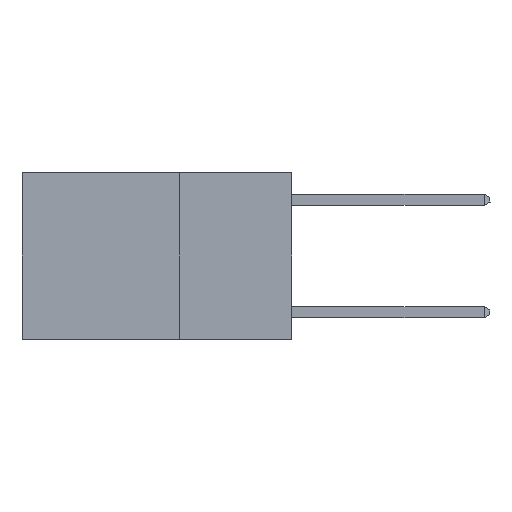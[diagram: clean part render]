
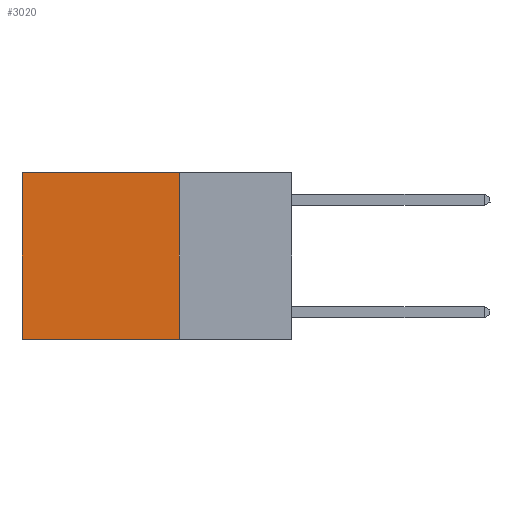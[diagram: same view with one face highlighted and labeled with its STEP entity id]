
A CAD part, left-side view. The second image highlights one B-rep face of the part: STEP entity #3020.
In plain terms, the highlighted planar face has unit normal (-1, 0, 0).
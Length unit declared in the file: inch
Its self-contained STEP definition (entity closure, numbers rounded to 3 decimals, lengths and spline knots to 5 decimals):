
#401 = EDGE_CURVE ( 'NONE', #8646, #3516, #3455, .T. ) ;
#670 = ORIENTED_EDGE ( 'NONE', *, *, #8644, .F. ) ;
#1688 = ORIENTED_EDGE ( 'NONE', *, *, #6867, .F. ) ;
#1991 = DIRECTION ( 'NONE',  ( 0., 1., 0. ) ) ;
#2136 = LINE ( 'NONE', #8721, #4109 ) ;
#2543 = DIRECTION ( 'NONE',  ( 0., 1., 0. ) ) ;
#3020 = ADVANCED_FACE ( 'NONE', ( #8531 ), #8884, .F. ) ;
#3200 = VECTOR ( 'NONE', #3690, 39.37008 ) ;
#3455 = LINE ( 'NONE', #4082, #3200 ) ;
#3516 = VERTEX_POINT ( 'NONE', #9144 ) ;
#3690 = DIRECTION ( 'NONE',  ( 0., 0., -1. ) ) ;
#3838 = ORIENTED_EDGE ( 'NONE', *, *, #5899, .T. ) ;
#3918 = ORIENTED_EDGE ( 'NONE', *, *, #401, .T. ) ;
#4082 = CARTESIAN_POINT ( 'NONE',  ( 0.2625, 0.6, 0. ) ) ;
#4109 = VECTOR ( 'NONE', #1991, 39.37008 ) ;
#4309 = LINE ( 'NONE', #10726, #6837 ) ;
#5013 = CARTESIAN_POINT ( 'NONE',  ( 0.2625, 0.25, 0. ) ) ;
#5429 = AXIS2_PLACEMENT_3D ( 'NONE', #7578, #8423, #7792 ) ;
#5561 = VERTEX_POINT ( 'NONE', #8742 ) ;
#5770 = DIRECTION ( 'NONE',  ( 0., 0., -1. ) ) ;
#5899 = EDGE_CURVE ( 'NONE', #5561, #8646, #10744, .T. ) ;
#6837 = VECTOR ( 'NONE', #5770, 39.37008 ) ;
#6867 = EDGE_CURVE ( 'NONE', #9092, #3516, #2136, .T. ) ;
#7578 = CARTESIAN_POINT ( 'NONE',  ( 0.2625, 0.25, 0. ) ) ;
#7792 = DIRECTION ( 'NONE',  ( 0., 0., -1. ) ) ;
#8339 = VECTOR ( 'NONE', #2543, 39.37008 ) ;
#8399 = EDGE_LOOP ( 'NONE', ( #3918, #1688, #670, #3838 ) ) ;
#8423 = DIRECTION ( 'NONE',  ( 1., 0., 0. ) ) ;
#8531 = FACE_OUTER_BOUND ( 'NONE', #8399, .T. ) ;
#8644 = EDGE_CURVE ( 'NONE', #5561, #9092, #4309, .T. ) ;
#8646 = VERTEX_POINT ( 'NONE', #9946 ) ;
#8721 = CARTESIAN_POINT ( 'NONE',  ( 0.2625, 0.25, -0.37 ) ) ;
#8742 = CARTESIAN_POINT ( 'NONE',  ( 0.2625, 0.25, 0. ) ) ;
#8884 = PLANE ( 'NONE',  #5429 ) ;
#9092 = VERTEX_POINT ( 'NONE', #10414 ) ;
#9144 = CARTESIAN_POINT ( 'NONE',  ( 0.2625, 0.6, -0.37 ) ) ;
#9946 = CARTESIAN_POINT ( 'NONE',  ( 0.2625, 0.6, 0. ) ) ;
#10414 = CARTESIAN_POINT ( 'NONE',  ( 0.2625, 0.25, -0.37 ) ) ;
#10726 = CARTESIAN_POINT ( 'NONE',  ( 0.2625, 0.25, 0. ) ) ;
#10744 = LINE ( 'NONE', #5013, #8339 ) ;
